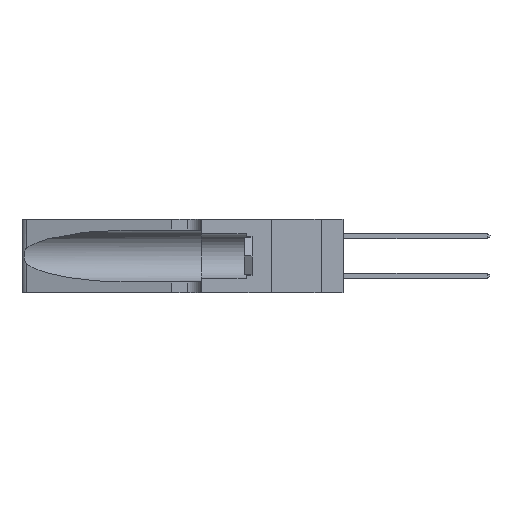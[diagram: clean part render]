
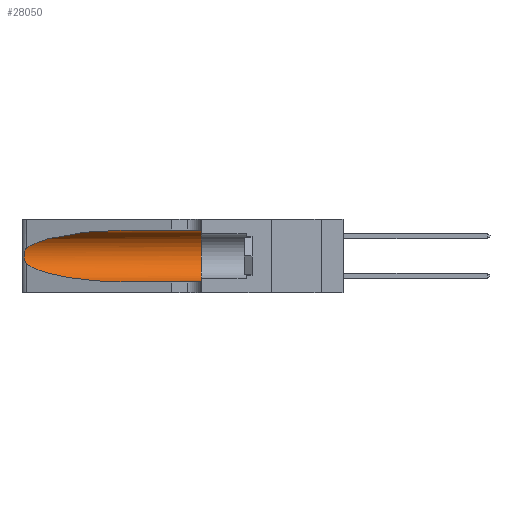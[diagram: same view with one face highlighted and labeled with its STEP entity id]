
A CAD part, left-side view. The second image highlights one B-rep face of the part: STEP entity #28050.
In plain terms, the highlighted cylindrical face has radius 3.308 mm (diameter 6.617 mm), a partial arc.
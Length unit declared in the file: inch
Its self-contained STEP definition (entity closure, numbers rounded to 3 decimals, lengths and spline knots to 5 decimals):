
#111 = B_SPLINE_CURVE_WITH_KNOTS ( 'NONE', 3,
 ( #21432, #27796, #24596, #18247, #40420, #34047, #30984, #12035, #40549, #21559, #37352, #21167, #14944, #18508 ),
 .UNSPECIFIED., .F., .F.,
 ( 4, 2, 2, 2, 2, 2, 4 ),
 ( 0., 0.00027, 0.00053, 0.00107, 0.0016, 0.00187, 0.00214 ),
 .UNSPECIFIED. ) ;
#891 = CARTESIAN_POINT ( 'NONE',  ( 0.25487, 1.22718, 0.22369 ) ) ;
#1647 = CARTESIAN_POINT ( 'NONE',  ( 0.1305, 0.35, 0.05475 ) ) ;
#1864 = CARTESIAN_POINT ( 'NONE',  ( 0.1305, 0.35, 0.31525 ) ) ;
#3367 = DIRECTION ( 'NONE',  ( 0., -1., 0. ) ) ;
#4396 = CARTESIAN_POINT ( 'NONE',  ( 0.2373, 1.15595, 0.08982 ) ) ;
#4457 = VERTEX_POINT ( 'NONE', #15875 ) ;
#5249 = CARTESIAN_POINT ( 'NONE',  ( 0.1305, 0.35, 0.185 ) ) ;
#6643 = CARTESIAN_POINT ( 'NONE',  ( 0.1305, 0.72297, 0.31525 ) ) ;
#6713 = CARTESIAN_POINT ( 'NONE',  ( 0.1305, 0.72297, 0.05475 ) ) ;
#7547 = CARTESIAN_POINT ( 'NONE',  ( 0.25487, 1.22718, 0.14631 ) ) ;
#7956 =( BOUNDED_CURVE ( )  B_SPLINE_CURVE ( 3, ( #7547, #4396, #13631, #14060 ),
 .UNSPECIFIED., .F., .F. ) 
 B_SPLINE_CURVE_WITH_KNOTS ( ( 4, 4 ),
 ( 3.44316, 4.71239 ),
 .UNSPECIFIED. ) 
 CURVE ( )  GEOMETRIC_REPRESENTATION_ITEM ( )  RATIONAL_B_SPLINE_CURVE ( ( 1., 0.87, 0.87, 1. ) ) 
 REPRESENTATION_ITEM ( '' )  );
#8286 = ORIENTED_EDGE ( 'NONE', *, *, #26529, .T. ) ;
#8432 = DIRECTION ( 'NONE',  ( 0., 0., 1. ) ) ;
#9102 = EDGE_LOOP ( 'NONE', ( #37379, #8286, #13232, #14927, #20573, #22000 ) ) ;
#9108 = CARTESIAN_POINT ( 'NONE',  ( 0.1305, 1.61858, 0.185 ) ) ;
#9699 = CYLINDRICAL_SURFACE ( 'NONE', #21958, 0.13025 ) ;
#10251 = CARTESIAN_POINT ( 'NONE',  ( 0.2373, 1.15595, 0.28018 ) ) ;
#10914 = VERTEX_POINT ( 'NONE', #1864 ) ;
#12035 = CARTESIAN_POINT ( 'NONE',  ( 0.26075, 1.23896, 0.178 ) ) ;
#12794 = EDGE_CURVE ( 'NONE', #23267, #10914, #27938, .T. ) ;
#13232 = ORIENTED_EDGE ( 'NONE', *, *, #27150, .T. ) ;
#13631 = CARTESIAN_POINT ( 'NONE',  ( 0.18966, 0.96281, 0.05475 ) ) ;
#14060 = CARTESIAN_POINT ( 'NONE',  ( 0.1305, 0.72297, 0.05475 ) ) ;
#14178 = FACE_OUTER_BOUND ( 'NONE', #9102, .T. ) ;
#14927 = ORIENTED_EDGE ( 'NONE', *, *, #35428, .T. ) ;
#14944 = CARTESIAN_POINT ( 'NONE',  ( 0.25555, 1.22993, 0.14849 ) ) ;
#15194 = DIRECTION ( 'NONE',  ( 0., -1., 0. ) ) ;
#15219 = CIRCLE ( 'NONE', #16566, 0.13025 ) ;
#15875 = CARTESIAN_POINT ( 'NONE',  ( 0.25487, 1.22718, 0.14631 ) ) ;
#16566 = AXIS2_PLACEMENT_3D ( 'NONE', #5249, #27383, #8432 ) ;
#18247 = CARTESIAN_POINT ( 'NONE',  ( 0.25787, 1.23484, 0.2124 ) ) ;
#18508 = CARTESIAN_POINT ( 'NONE',  ( 0.25487, 1.22718, 0.14631 ) ) ;
#19500 = VECTOR ( 'NONE', #3367, 39.37008 ) ;
#19987 = VERTEX_POINT ( 'NONE', #35431 ) ;
#20573 = ORIENTED_EDGE ( 'NONE', *, *, #36638, .F. ) ;
#20788 = LINE ( 'NONE', #22164, #25199 ) ;
#21167 = CARTESIAN_POINT ( 'NONE',  ( 0.25639, 1.23186, 0.15144 ) ) ;
#21432 = CARTESIAN_POINT ( 'NONE',  ( 0.25487, 1.22718, 0.22369 ) ) ;
#21559 = CARTESIAN_POINT ( 'NONE',  ( 0.25856, 1.23593, 0.16098 ) ) ;
#21891 = CARTESIAN_POINT ( 'NONE',  ( 0.1305, 1.61858, 0.31525 ) ) ;
#21958 = AXIS2_PLACEMENT_3D ( 'NONE', #9108, #15194, #34438 ) ;
#22000 = ORIENTED_EDGE ( 'NONE', *, *, #12794, .F. ) ;
#22164 = CARTESIAN_POINT ( 'NONE',  ( 0.1305, 1.61858, 0.05475 ) ) ;
#22444 = DIRECTION ( 'NONE',  ( 0., -1., 0. ) ) ;
#23267 = VERTEX_POINT ( 'NONE', #6643 ) ;
#24596 = CARTESIAN_POINT ( 'NONE',  ( 0.25639, 1.23184, 0.21858 ) ) ;
#25199 = VECTOR ( 'NONE', #22444, 39.37008 ) ;
#26279 = CARTESIAN_POINT ( 'NONE',  ( 0.18966, 0.96281, 0.31525 ) ) ;
#26529 = EDGE_CURVE ( 'NONE', #19987, #4457, #111, .T. ) ;
#26710 = CARTESIAN_POINT ( 'NONE',  ( 0.1305, 0.72297, 0.31525 ) ) ;
#27150 = EDGE_CURVE ( 'NONE', #4457, #36804, #7956, .T. ) ;
#27383 = DIRECTION ( 'NONE',  ( 0., 1., 0. ) ) ;
#27796 = CARTESIAN_POINT ( 'NONE',  ( 0.25555, 1.22994, 0.2215 ) ) ;
#27938 = LINE ( 'NONE', #21891, #19500 ) ;
#28050 = ADVANCED_FACE ( 'NONE', ( #14178 ), #9699, .F. ) ;
#30984 = CARTESIAN_POINT ( 'NONE',  ( 0.26075, 1.23896, 0.19203 ) ) ;
#34047 = CARTESIAN_POINT ( 'NONE',  ( 0.26018, 1.23835, 0.19895 ) ) ;
#34364 = EDGE_CURVE ( 'NONE', #23267, #19987, #35608, .T. ) ;
#34438 = DIRECTION ( 'NONE',  ( 0., 0., -1. ) ) ;
#35428 = EDGE_CURVE ( 'NONE', #36804, #39346, #20788, .T. ) ;
#35431 = CARTESIAN_POINT ( 'NONE',  ( 0.25487, 1.22718, 0.22369 ) ) ;
#35608 =( BOUNDED_CURVE ( )  B_SPLINE_CURVE ( 3, ( #26710, #26279, #10251, #891 ),
 .UNSPECIFIED., .F., .T. ) 
 B_SPLINE_CURVE_WITH_KNOTS ( ( 4, 4 ),
 ( 1.5708, 2.84003 ),
 .UNSPECIFIED. ) 
 CURVE ( )  GEOMETRIC_REPRESENTATION_ITEM ( )  RATIONAL_B_SPLINE_CURVE ( ( 1., 0.87, 0.87, 1. ) ) 
 REPRESENTATION_ITEM ( '' )  );
#36638 = EDGE_CURVE ( 'NONE', #10914, #39346, #15219, .T. ) ;
#36804 = VERTEX_POINT ( 'NONE', #6713 ) ;
#37352 = CARTESIAN_POINT ( 'NONE',  ( 0.25789, 1.23486, 0.15765 ) ) ;
#37379 = ORIENTED_EDGE ( 'NONE', *, *, #34364, .T. ) ;
#39346 = VERTEX_POINT ( 'NONE', #1647 ) ;
#40420 = CARTESIAN_POINT ( 'NONE',  ( 0.25854, 1.2359, 0.20912 ) ) ;
#40549 = CARTESIAN_POINT ( 'NONE',  ( 0.26017, 1.23833, 0.17102 ) ) ;
